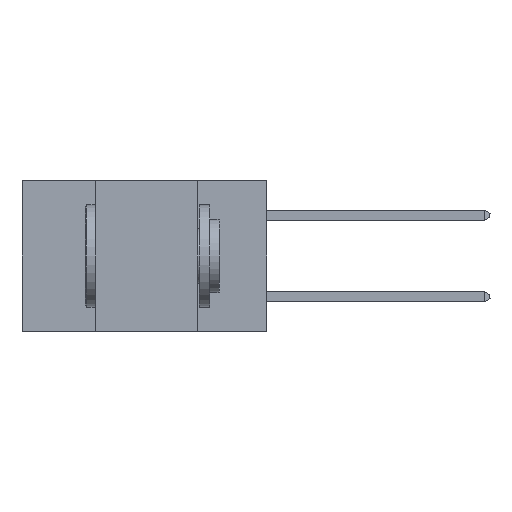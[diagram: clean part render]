
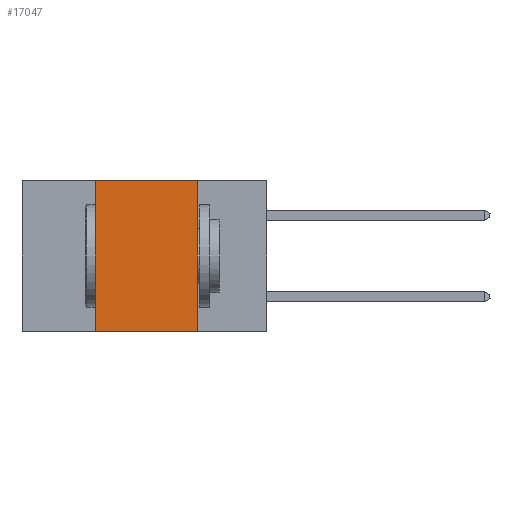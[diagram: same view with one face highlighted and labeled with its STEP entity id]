
A CAD part, left-side view. The second image highlights one B-rep face of the part: STEP entity #17047.
In plain terms, the highlighted planar face has unit normal (-1, 0, 0).
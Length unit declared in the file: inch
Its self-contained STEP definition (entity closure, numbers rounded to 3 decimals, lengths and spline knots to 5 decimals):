
#514 = EDGE_CURVE ( 'NONE', #21689, #19403, #38648, .T. ) ;
#1493 = VECTOR ( 'NONE', #33169, 39.37008 ) ;
#1916 = DIRECTION ( 'NONE',  ( 0., -1., 0. ) ) ;
#2156 = ORIENTED_EDGE ( 'NONE', *, *, #15618, .F. ) ;
#6106 = ORIENTED_EDGE ( 'NONE', *, *, #33217, .T. ) ;
#6189 = VECTOR ( 'NONE', #11163, 39.37008 ) ;
#8680 = CARTESIAN_POINT ( 'NONE',  ( 0., 0.17, 0. ) ) ;
#9860 = PLANE ( 'NONE',  #21850 ) ;
#11030 = LINE ( 'NONE', #11811, #11999 ) ;
#11163 = DIRECTION ( 'NONE',  ( 0., -1., 0. ) ) ;
#11297 = CARTESIAN_POINT ( 'NONE',  ( 0., 0.6, 0. ) ) ;
#11811 = CARTESIAN_POINT ( 'NONE',  ( 0., 0.42, 0. ) ) ;
#11999 = VECTOR ( 'NONE', #30235, 39.37008 ) ;
#12925 = VERTEX_POINT ( 'NONE', #25851 ) ;
#12998 = DIRECTION ( 'NONE',  ( 1., 0., 0. ) ) ;
#15618 = EDGE_CURVE ( 'NONE', #19403, #12925, #26247, .T. ) ;
#17047 = ADVANCED_FACE ( 'NONE', ( #20790 ), #9860, .F. ) ;
#19403 = VERTEX_POINT ( 'NONE', #38580 ) ;
#20510 = CARTESIAN_POINT ( 'NONE',  ( 0., 0.6, -0.37 ) ) ;
#20623 = ORIENTED_EDGE ( 'NONE', *, *, #35223, .F. ) ;
#20790 = FACE_OUTER_BOUND ( 'NONE', #23838, .T. ) ;
#20883 = CARTESIAN_POINT ( 'NONE',  ( 0., 0.42, -0.37 ) ) ;
#21689 = VERTEX_POINT ( 'NONE', #30156 ) ;
#21850 = AXIS2_PLACEMENT_3D ( 'NONE', #31328, #12998, #34326 ) ;
#22318 = VERTEX_POINT ( 'NONE', #20883 ) ;
#23838 = EDGE_LOOP ( 'NONE', ( #2156, #26889, #20623, #6106 ) ) ;
#25851 = CARTESIAN_POINT ( 'NONE',  ( 0., 0.17, -0.37 ) ) ;
#26247 = LINE ( 'NONE', #8680, #1493 ) ;
#26889 = ORIENTED_EDGE ( 'NONE', *, *, #514, .F. ) ;
#29028 = VECTOR ( 'NONE', #1916, 39.37008 ) ;
#30156 = CARTESIAN_POINT ( 'NONE',  ( 0., 0.42, 0. ) ) ;
#30235 = DIRECTION ( 'NONE',  ( 0., 0., 1. ) ) ;
#31328 = CARTESIAN_POINT ( 'NONE',  ( 0., 0.6, 0. ) ) ;
#33169 = DIRECTION ( 'NONE',  ( 0., 0., -1. ) ) ;
#33217 = EDGE_CURVE ( 'NONE', #22318, #12925, #36960, .T. ) ;
#34326 = DIRECTION ( 'NONE',  ( 0., 0., -1. ) ) ;
#35223 = EDGE_CURVE ( 'NONE', #22318, #21689, #11030, .T. ) ;
#36960 = LINE ( 'NONE', #20510, #29028 ) ;
#38580 = CARTESIAN_POINT ( 'NONE',  ( 0., 0.17, 0. ) ) ;
#38648 = LINE ( 'NONE', #11297, #6189 ) ;
